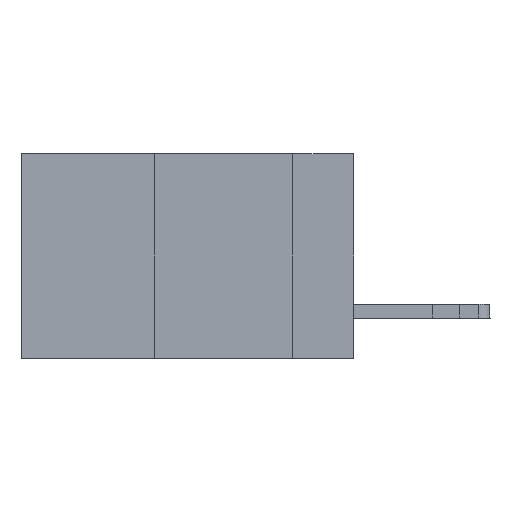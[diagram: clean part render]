
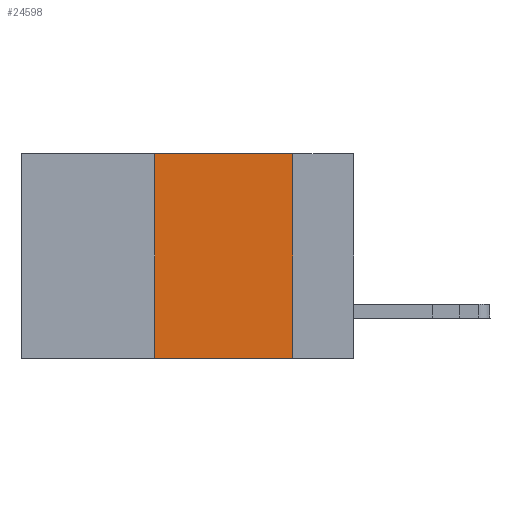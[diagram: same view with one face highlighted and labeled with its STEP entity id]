
A CAD part, left-side view. The second image highlights one B-rep face of the part: STEP entity #24598.
In plain terms, the highlighted planar face has unit normal (-1, 0, 0).
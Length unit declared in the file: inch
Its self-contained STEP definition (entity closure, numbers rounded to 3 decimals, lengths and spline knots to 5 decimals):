
#585 = EDGE_CURVE ( 'NONE', #13206, #7654, #11442, .T. ) ;
#1423 = VERTEX_POINT ( 'NONE', #1520 ) ;
#1520 = CARTESIAN_POINT ( 'NONE',  ( 0., 0.11, -0.37 ) ) ;
#3608 = ORIENTED_EDGE ( 'NONE', *, *, #15240, .F. ) ;
#3886 = DIRECTION ( 'NONE',  ( 0., -1., 0. ) ) ;
#3929 = CARTESIAN_POINT ( 'NONE',  ( 0., 0.36, 0. ) ) ;
#3945 = VECTOR ( 'NONE', #10088, 39.37008 ) ;
#4518 = DIRECTION ( 'NONE',  ( 1., 0., 0. ) ) ;
#4593 = CARTESIAN_POINT ( 'NONE',  ( 0., 0.11, 0. ) ) ;
#4605 = LINE ( 'NONE', #24374, #3945 ) ;
#5009 = CARTESIAN_POINT ( 'NONE',  ( 0., 0.36, -0.37 ) ) ;
#5429 = ORIENTED_EDGE ( 'NONE', *, *, #15553, .T. ) ;
#6200 = VECTOR ( 'NONE', #13222, 39.37008 ) ;
#6538 = ORIENTED_EDGE ( 'NONE', *, *, #17515, .F. ) ;
#6569 = VECTOR ( 'NONE', #15093, 39.37008 ) ;
#7165 = VERTEX_POINT ( 'NONE', #4593 ) ;
#7654 = VERTEX_POINT ( 'NONE', #3929 ) ;
#10088 = DIRECTION ( 'NONE',  ( 0., -1., 0. ) ) ;
#11442 = LINE ( 'NONE', #15114, #6569 ) ;
#12764 = PLANE ( 'NONE',  #25836 ) ;
#13206 = VERTEX_POINT ( 'NONE', #5009 ) ;
#13222 = DIRECTION ( 'NONE',  ( 0., 0., -1. ) ) ;
#15093 = DIRECTION ( 'NONE',  ( 0., 0., 1. ) ) ;
#15114 = CARTESIAN_POINT ( 'NONE',  ( 0., 0.36, 0. ) ) ;
#15240 = EDGE_CURVE ( 'NONE', #7165, #1423, #22763, .T. ) ;
#15553 = EDGE_CURVE ( 'NONE', #13206, #1423, #4605, .T. ) ;
#16470 = FACE_OUTER_BOUND ( 'NONE', #20693, .T. ) ;
#16777 = ORIENTED_EDGE ( 'NONE', *, *, #585, .F. ) ;
#16975 = CARTESIAN_POINT ( 'NONE',  ( 0., 0.6, 0. ) ) ;
#17209 = VECTOR ( 'NONE', #3886, 39.37008 ) ;
#17515 = EDGE_CURVE ( 'NONE', #7654, #7165, #17856, .T. ) ;
#17856 = LINE ( 'NONE', #20512, #17209 ) ;
#19063 = DIRECTION ( 'NONE',  ( 0., 0., -1. ) ) ;
#20512 = CARTESIAN_POINT ( 'NONE',  ( 0., 0.6, 0. ) ) ;
#20693 = EDGE_LOOP ( 'NONE', ( #3608, #6538, #16777, #5429 ) ) ;
#22763 = LINE ( 'NONE', #23526, #6200 ) ;
#23526 = CARTESIAN_POINT ( 'NONE',  ( 0., 0.11, 0. ) ) ;
#24374 = CARTESIAN_POINT ( 'NONE',  ( 0., 0.6, -0.37 ) ) ;
#24598 = ADVANCED_FACE ( 'NONE', ( #16470 ), #12764, .F. ) ;
#25836 = AXIS2_PLACEMENT_3D ( 'NONE', #16975, #4518, #19063 ) ;
